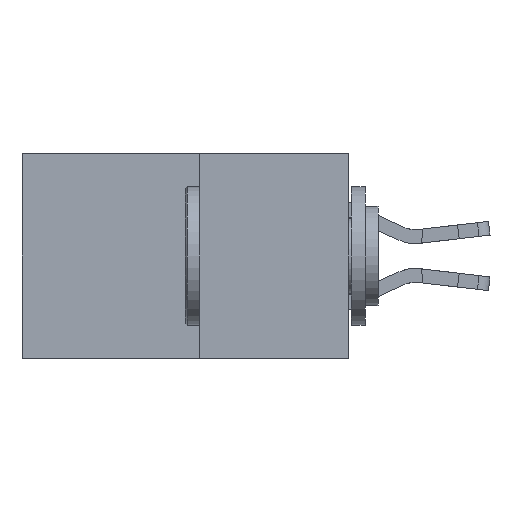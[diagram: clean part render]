
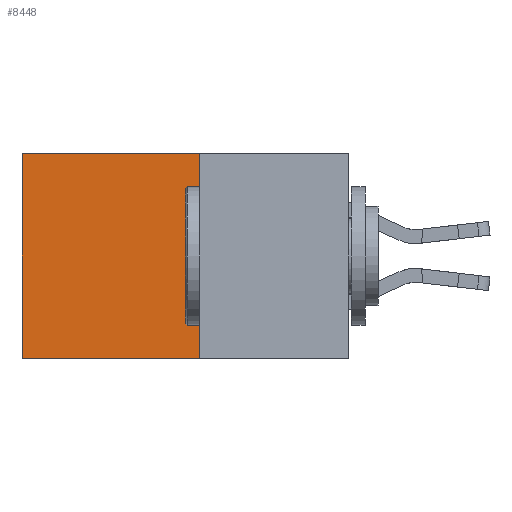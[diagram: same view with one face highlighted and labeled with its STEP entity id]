
A CAD part, left-side view. The second image highlights one B-rep face of the part: STEP entity #8448.
In plain terms, the highlighted planar face has unit normal (-1, 0, 0).
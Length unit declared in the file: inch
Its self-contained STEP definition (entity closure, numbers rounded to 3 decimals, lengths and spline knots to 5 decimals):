
#895 = ORIENTED_EDGE ( 'NONE', *, *, #4289, .T. ) ;
#1322 = CARTESIAN_POINT ( 'NONE',  ( 0.277, 0.27, -0.37 ) ) ;
#2144 = DIRECTION ( 'NONE',  ( 0., 0., -1. ) ) ;
#2490 = CARTESIAN_POINT ( 'NONE',  ( 0.277, 0.27, -0.37 ) ) ;
#2772 = EDGE_LOOP ( 'NONE', ( #895, #4534, #7857, #14154 ) ) ;
#2905 = AXIS2_PLACEMENT_3D ( 'NONE', #2490, #3715, #12270 ) ;
#3039 = CARTESIAN_POINT ( 'NONE',  ( 0.277, 0.59, 0. ) ) ;
#3641 = LINE ( 'NONE', #9498, #9809 ) ;
#3715 = DIRECTION ( 'NONE',  ( 1., 0., 0. ) ) ;
#4091 = CARTESIAN_POINT ( 'NONE',  ( 0.277, 0.27, 0. ) ) ;
#4190 = DIRECTION ( 'NONE',  ( 0., 1., 0. ) ) ;
#4289 = EDGE_CURVE ( 'NONE', #10932, #9874, #6445, .T. ) ;
#4532 = LINE ( 'NONE', #1322, #4932 ) ;
#4534 = ORIENTED_EDGE ( 'NONE', *, *, #10672, .F. ) ;
#4569 = VERTEX_POINT ( 'NONE', #10368 ) ;
#4920 = PLANE ( 'NONE',  #2905 ) ;
#4932 = VECTOR ( 'NONE', #11106, 39.37008 ) ;
#5195 = CARTESIAN_POINT ( 'NONE',  ( 0.277, 0.59, -0.37 ) ) ;
#5315 = CARTESIAN_POINT ( 'NONE',  ( 0.277, 0.59, -0.37 ) ) ;
#6445 = LINE ( 'NONE', #5195, #10040 ) ;
#6987 = VECTOR ( 'NONE', #4190, 39.37008 ) ;
#7264 = EDGE_CURVE ( 'NONE', #7534, #10932, #13353, .T. ) ;
#7534 = VERTEX_POINT ( 'NONE', #10764 ) ;
#7857 = ORIENTED_EDGE ( 'NONE', *, *, #8199, .F. ) ;
#8199 = EDGE_CURVE ( 'NONE', #7534, #4569, #3641, .T. ) ;
#8448 = ADVANCED_FACE ( 'NONE', ( #12785 ), #4920, .F. ) ;
#9498 = CARTESIAN_POINT ( 'NONE',  ( 0.277, 0.27, -0.37 ) ) ;
#9809 = VECTOR ( 'NONE', #2144, 39.37008 ) ;
#9874 = VERTEX_POINT ( 'NONE', #5315 ) ;
#10040 = VECTOR ( 'NONE', #14642, 39.37008 ) ;
#10368 = CARTESIAN_POINT ( 'NONE',  ( 0.277, 0.27, -0.37 ) ) ;
#10672 = EDGE_CURVE ( 'NONE', #4569, #9874, #4532, .T. ) ;
#10764 = CARTESIAN_POINT ( 'NONE',  ( 0.277, 0.27, 0. ) ) ;
#10932 = VERTEX_POINT ( 'NONE', #3039 ) ;
#11106 = DIRECTION ( 'NONE',  ( 0., 1., 0. ) ) ;
#12270 = DIRECTION ( 'NONE',  ( 0., 0., -1. ) ) ;
#12785 = FACE_OUTER_BOUND ( 'NONE', #2772, .T. ) ;
#13353 = LINE ( 'NONE', #4091, #6987 ) ;
#14154 = ORIENTED_EDGE ( 'NONE', *, *, #7264, .T. ) ;
#14642 = DIRECTION ( 'NONE',  ( 0., 0., -1. ) ) ;
